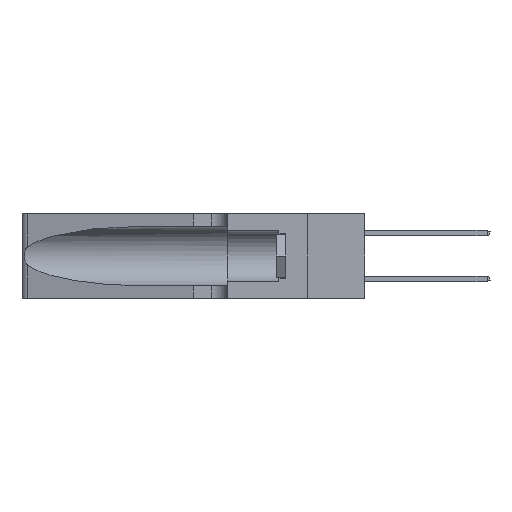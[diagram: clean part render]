
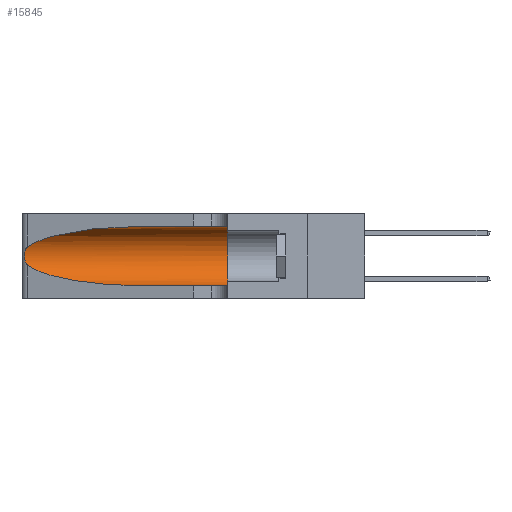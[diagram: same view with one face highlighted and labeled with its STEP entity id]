
A CAD part, left-side view. The second image highlights one B-rep face of the part: STEP entity #15845.
In plain terms, the highlighted cylindrical face has radius 3.308 mm (diameter 6.617 mm), a partial arc.
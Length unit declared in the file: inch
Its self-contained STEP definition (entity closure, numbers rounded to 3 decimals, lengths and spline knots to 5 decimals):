
#128 = ORIENTED_EDGE ( 'NONE', *, *, #2686, .T. ) ;
#677 = CARTESIAN_POINT ( 'NONE',  ( 0.1305, 0.72297, 0.05475 ) ) ;
#1888 = VECTOR ( 'NONE', #20765, 39.37008 ) ;
#1915 = CARTESIAN_POINT ( 'NONE',  ( 0.1305, 0.72297, 0.31525 ) ) ;
#2302 =( BOUNDED_CURVE ( )  B_SPLINE_CURVE ( 3, ( #1915, #3420, #17146, #20580 ),
 .UNSPECIFIED., .F., .F. ) 
 B_SPLINE_CURVE_WITH_KNOTS ( ( 4, 4 ),
 ( 1.5708, 2.84003 ),
 .UNSPECIFIED. ) 
 CURVE ( )  GEOMETRIC_REPRESENTATION_ITEM ( )  RATIONAL_B_SPLINE_CURVE ( ( 1., 0.87, 0.87, 1. ) ) 
 REPRESENTATION_ITEM ( '' )  );
#2568 = B_SPLINE_CURVE_WITH_KNOTS ( 'NONE', 3,
 ( #20922, #10748, #14155, #6306, #20022, #17703, #7039, #16022, #16985, #7172, #3848, #17844, #7735, #4221 ),
 .UNSPECIFIED., .F., .F.,
 ( 4, 2, 2, 2, 2, 2, 4 ),
 ( 0., 0.00027, 0.00053, 0.00107, 0.0016, 0.00187, 0.00214 ),
 .UNSPECIFIED. ) ;
#2603 = EDGE_CURVE ( 'NONE', #19285, #13233, #21203, .T. ) ;
#2686 = EDGE_CURVE ( 'NONE', #17546, #10691, #2568, .T. ) ;
#2959 = VERTEX_POINT ( 'NONE', #4389 ) ;
#3358 = CARTESIAN_POINT ( 'NONE',  ( 0.25487, 1.22718, 0.22369 ) ) ;
#3420 = CARTESIAN_POINT ( 'NONE',  ( 0.18966, 0.96281, 0.31525 ) ) ;
#3848 = CARTESIAN_POINT ( 'NONE',  ( 0.25789, 1.23486, 0.15765 ) ) ;
#4221 = CARTESIAN_POINT ( 'NONE',  ( 0.25487, 1.22718, 0.14631 ) ) ;
#4389 = CARTESIAN_POINT ( 'NONE',  ( 0.1305, 0.72297, 0.05475 ) ) ;
#4976 = CARTESIAN_POINT ( 'NONE',  ( 0.1305, 1.61858, 0.185 ) ) ;
#5851 = EDGE_LOOP ( 'NONE', ( #11571, #128, #17561, #21948, #21897, #14116 ) ) ;
#6282 =( BOUNDED_CURVE ( )  B_SPLINE_CURVE ( 3, ( #7303, #15986, #19561, #677 ),
 .UNSPECIFIED., .F., .F. ) 
 B_SPLINE_CURVE_WITH_KNOTS ( ( 4, 4 ),
 ( 3.44316, 4.71239 ),
 .UNSPECIFIED. ) 
 CURVE ( )  GEOMETRIC_REPRESENTATION_ITEM ( )  RATIONAL_B_SPLINE_CURVE ( ( 1., 0.87, 0.87, 1. ) ) 
 REPRESENTATION_ITEM ( '' )  );
#6306 = CARTESIAN_POINT ( 'NONE',  ( 0.25787, 1.23484, 0.2124 ) ) ;
#6664 = DIRECTION ( 'NONE',  ( 0., 0., 1. ) ) ;
#6856 = DIRECTION ( 'NONE',  ( 0., 0., -1. ) ) ;
#7039 = CARTESIAN_POINT ( 'NONE',  ( 0.26075, 1.23896, 0.19203 ) ) ;
#7172 = CARTESIAN_POINT ( 'NONE',  ( 0.25856, 1.23593, 0.16098 ) ) ;
#7303 = CARTESIAN_POINT ( 'NONE',  ( 0.25487, 1.22718, 0.14631 ) ) ;
#7601 = VERTEX_POINT ( 'NONE', #21095 ) ;
#7735 = CARTESIAN_POINT ( 'NONE',  ( 0.25555, 1.22993, 0.14849 ) ) ;
#8458 = DIRECTION ( 'NONE',  ( 0., 1., 0. ) ) ;
#9376 = AXIS2_PLACEMENT_3D ( 'NONE', #4976, #13693, #6856 ) ;
#9621 = CARTESIAN_POINT ( 'NONE',  ( 0.25487, 1.22718, 0.14631 ) ) ;
#10691 = VERTEX_POINT ( 'NONE', #9621 ) ;
#10748 = CARTESIAN_POINT ( 'NONE',  ( 0.25555, 1.22994, 0.2215 ) ) ;
#11571 = ORIENTED_EDGE ( 'NONE', *, *, #18168, .T. ) ;
#11827 = CARTESIAN_POINT ( 'NONE',  ( 0.1305, 1.61858, 0.05475 ) ) ;
#12001 = CARTESIAN_POINT ( 'NONE',  ( 0.1305, 0.72297, 0.31525 ) ) ;
#13233 = VERTEX_POINT ( 'NONE', #21124 ) ;
#13413 = EDGE_CURVE ( 'NONE', #2959, #7601, #15587, .T. ) ;
#13693 = DIRECTION ( 'NONE',  ( 0., -1., 0. ) ) ;
#14116 = ORIENTED_EDGE ( 'NONE', *, *, #2603, .F. ) ;
#14155 = CARTESIAN_POINT ( 'NONE',  ( 0.25639, 1.23184, 0.21858 ) ) ;
#14794 = CYLINDRICAL_SURFACE ( 'NONE', #9376, 0.13025 ) ;
#15295 = DIRECTION ( 'NONE',  ( 0., -1., 0. ) ) ;
#15587 = LINE ( 'NONE', #11827, #20645 ) ;
#15845 = ADVANCED_FACE ( 'NONE', ( #18228 ), #14794, .F. ) ;
#15986 = CARTESIAN_POINT ( 'NONE',  ( 0.2373, 1.15595, 0.08982 ) ) ;
#16022 = CARTESIAN_POINT ( 'NONE',  ( 0.26075, 1.23896, 0.178 ) ) ;
#16985 = CARTESIAN_POINT ( 'NONE',  ( 0.26017, 1.23833, 0.17102 ) ) ;
#17078 = CARTESIAN_POINT ( 'NONE',  ( 0.1305, 0.35, 0.185 ) ) ;
#17146 = CARTESIAN_POINT ( 'NONE',  ( 0.2373, 1.15595, 0.28018 ) ) ;
#17546 = VERTEX_POINT ( 'NONE', #3358 ) ;
#17561 = ORIENTED_EDGE ( 'NONE', *, *, #18995, .T. ) ;
#17703 = CARTESIAN_POINT ( 'NONE',  ( 0.26018, 1.23835, 0.19895 ) ) ;
#17844 = CARTESIAN_POINT ( 'NONE',  ( 0.25639, 1.23186, 0.15144 ) ) ;
#18168 = EDGE_CURVE ( 'NONE', #19285, #17546, #2302, .T. ) ;
#18218 = CIRCLE ( 'NONE', #21313, 0.13025 ) ;
#18228 = FACE_OUTER_BOUND ( 'NONE', #5851, .T. ) ;
#18995 = EDGE_CURVE ( 'NONE', #10691, #2959, #6282, .T. ) ;
#19285 = VERTEX_POINT ( 'NONE', #12001 ) ;
#19561 = CARTESIAN_POINT ( 'NONE',  ( 0.18966, 0.96281, 0.05475 ) ) ;
#20022 = CARTESIAN_POINT ( 'NONE',  ( 0.25854, 1.2359, 0.20912 ) ) ;
#20580 = CARTESIAN_POINT ( 'NONE',  ( 0.25487, 1.22718, 0.22369 ) ) ;
#20645 = VECTOR ( 'NONE', #15295, 39.37008 ) ;
#20696 = CARTESIAN_POINT ( 'NONE',  ( 0.1305, 1.61858, 0.31525 ) ) ;
#20765 = DIRECTION ( 'NONE',  ( 0., -1., 0. ) ) ;
#20922 = CARTESIAN_POINT ( 'NONE',  ( 0.25487, 1.22718, 0.22369 ) ) ;
#21095 = CARTESIAN_POINT ( 'NONE',  ( 0.1305, 0.35, 0.05475 ) ) ;
#21124 = CARTESIAN_POINT ( 'NONE',  ( 0.1305, 0.35, 0.31525 ) ) ;
#21203 = LINE ( 'NONE', #20696, #1888 ) ;
#21313 = AXIS2_PLACEMENT_3D ( 'NONE', #17078, #8458, #6664 ) ;
#21897 = ORIENTED_EDGE ( 'NONE', *, *, #22022, .F. ) ;
#21948 = ORIENTED_EDGE ( 'NONE', *, *, #13413, .T. ) ;
#22022 = EDGE_CURVE ( 'NONE', #13233, #7601, #18218, .T. ) ;
